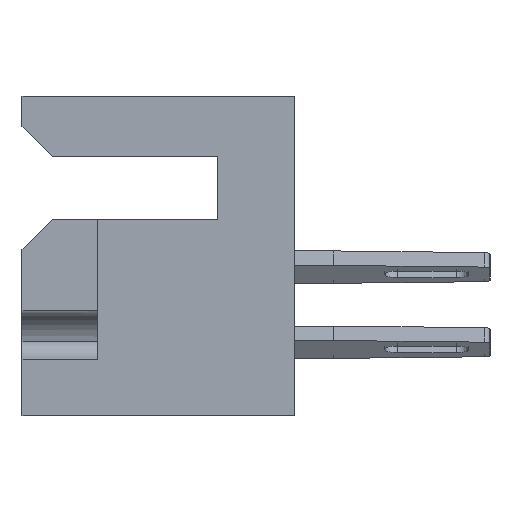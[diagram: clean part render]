
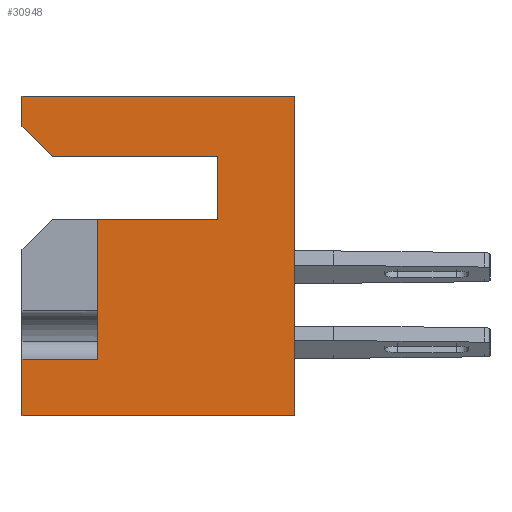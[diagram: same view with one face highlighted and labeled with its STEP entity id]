
A CAD part, left-side view. The second image highlights one B-rep face of the part: STEP entity #30948.
In plain terms, the highlighted planar face has unit normal (-1, 0, 0).
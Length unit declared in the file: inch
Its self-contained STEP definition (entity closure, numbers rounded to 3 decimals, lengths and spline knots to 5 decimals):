
#488 = EDGE_CURVE ( 'NONE', #5836, #26550, #2520, .T. ) ;
#700 = EDGE_CURVE ( 'NONE', #21298, #19477, #2494, .T. ) ;
#901 = LINE ( 'NONE', #11185, #5777 ) ;
#1414 = PLANE ( 'NONE',  #14213 ) ;
#1489 = DIRECTION ( 'NONE',  ( 0., 0., 1. ) ) ;
#1533 = ORIENTED_EDGE ( 'NONE', *, *, #700, .F. ) ;
#2153 = CARTESIAN_POINT ( 'NONE',  ( 0., 0.328, -0.205 ) ) ;
#2340 = DIRECTION ( 'NONE',  ( 0., 1., 0. ) ) ;
#2494 = LINE ( 'NONE', #4337, #11495 ) ;
#2520 = LINE ( 'NONE', #4237, #27203 ) ;
#3116 = CARTESIAN_POINT ( 'NONE',  ( 0., 0.128, -0.205 ) ) ;
#3589 = VERTEX_POINT ( 'NONE', #28175 ) ;
#4088 = CARTESIAN_POINT ( 'NONE',  ( 0., 0.453, 0. ) ) ;
#4125 = VERTEX_POINT ( 'NONE', #9381 ) ;
#4237 = CARTESIAN_POINT ( 'NONE',  ( 0., 0.128, -0.1 ) ) ;
#4260 = VECTOR ( 'NONE', #20819, 39.37008 ) ;
#4337 = CARTESIAN_POINT ( 'NONE',  ( 0., 0.453, 0. ) ) ;
#4658 = DIRECTION ( 'NONE',  ( 0., 0., 1. ) ) ;
#5777 = VECTOR ( 'NONE', #30473, 39.37008 ) ;
#5836 = VERTEX_POINT ( 'NONE', #18371 ) ;
#5914 = VERTEX_POINT ( 'NONE', #18853 ) ;
#6883 = LINE ( 'NONE', #22700, #22587 ) ;
#7056 = VECTOR ( 'NONE', #2340, 39.37008 ) ;
#7673 = EDGE_CURVE ( 'NONE', #17577, #4125, #25529, .T. ) ;
#8258 = ORIENTED_EDGE ( 'NONE', *, *, #13072, .F. ) ;
#8823 = ORIENTED_EDGE ( 'NONE', *, *, #28771, .T. ) ;
#9285 = EDGE_LOOP ( 'NONE', ( #25436, #1533, #11394, #15115, #19073, #30682, #8823, #24711, #25405, #24883, #8258 ) ) ;
#9306 = CARTESIAN_POINT ( 'NONE',  ( 0., 0.453, -0.437 ) ) ;
#9381 = CARTESIAN_POINT ( 'NONE',  ( 0., 0.453, 0. ) ) ;
#10070 = VECTOR ( 'NONE', #29678, 39.37008 ) ;
#10959 = DIRECTION ( 'NONE',  ( 0., 0., 1. ) ) ;
#11185 = CARTESIAN_POINT ( 'NONE',  ( 0., 0.328, -0.205 ) ) ;
#11394 = ORIENTED_EDGE ( 'NONE', *, *, #28670, .T. ) ;
#11495 = VECTOR ( 'NONE', #4658, 39.37008 ) ;
#11690 = EDGE_CURVE ( 'NONE', #26550, #3589, #13669, .T. ) ;
#12131 = VERTEX_POINT ( 'NONE', #26376 ) ;
#12239 = EDGE_CURVE ( 'NONE', #12131, #5914, #6883, .T. ) ;
#12410 = EDGE_CURVE ( 'NONE', #4125, #5914, #17750, .T. ) ;
#12455 = DIRECTION ( 'NONE',  ( 0., 0., 1. ) ) ;
#13072 = EDGE_CURVE ( 'NONE', #23057, #21686, #901, .T. ) ;
#13443 = CARTESIAN_POINT ( 'NONE',  ( 0., 0.453, 0. ) ) ;
#13669 = LINE ( 'NONE', #15216, #26010 ) ;
#14105 = EDGE_CURVE ( 'NONE', #5836, #21686, #23644, .T. ) ;
#14213 = AXIS2_PLACEMENT_3D ( 'NONE', #22846, #18183, #18483 ) ;
#15112 = DIRECTION ( 'NONE',  ( 0., 1., 0. ) ) ;
#15115 = ORIENTED_EDGE ( 'NONE', *, *, #12239, .T. ) ;
#15216 = CARTESIAN_POINT ( 'NONE',  ( 0., 0.128, -0.1 ) ) ;
#16727 = CARTESIAN_POINT ( 'NONE',  ( 0., 0.328, -0.437 ) ) ;
#17142 = LINE ( 'NONE', #18899, #7056 ) ;
#17577 = VERTEX_POINT ( 'NONE', #28411 ) ;
#17750 = LINE ( 'NONE', #4088, #4260 ) ;
#18183 = DIRECTION ( 'NONE',  ( 1., 0., 0. ) ) ;
#18371 = CARTESIAN_POINT ( 'NONE',  ( 0., 0.128, -0.205 ) ) ;
#18410 = CARTESIAN_POINT ( 'NONE',  ( 0., 0.403, -0.1 ) ) ;
#18483 = DIRECTION ( 'NONE',  ( 0., 0., -1. ) ) ;
#18853 = CARTESIAN_POINT ( 'NONE',  ( 0., 0., 0. ) ) ;
#18899 = CARTESIAN_POINT ( 'NONE',  ( 0., 0.328, -0.437 ) ) ;
#19073 = ORIENTED_EDGE ( 'NONE', *, *, #12410, .F. ) ;
#19477 = VERTEX_POINT ( 'NONE', #9306 ) ;
#20092 = CARTESIAN_POINT ( 'NONE',  ( 0., 0.453, -0.531 ) ) ;
#20819 = DIRECTION ( 'NONE',  ( 0., -1., 0. ) ) ;
#21298 = VERTEX_POINT ( 'NONE', #24364 ) ;
#21664 = LINE ( 'NONE', #20092, #10070 ) ;
#21686 = VERTEX_POINT ( 'NONE', #2153 ) ;
#22587 = VECTOR ( 'NONE', #12455, 39.37008 ) ;
#22700 = CARTESIAN_POINT ( 'NONE',  ( 0., 0., 0. ) ) ;
#22846 = CARTESIAN_POINT ( 'NONE',  ( 0., 0.453, 0. ) ) ;
#23057 = VERTEX_POINT ( 'NONE', #16727 ) ;
#23644 = LINE ( 'NONE', #3116, #28129 ) ;
#24364 = CARTESIAN_POINT ( 'NONE',  ( 0., 0.453, -0.531 ) ) ;
#24711 = ORIENTED_EDGE ( 'NONE', *, *, #11690, .F. ) ;
#24775 = DIRECTION ( 'NONE',  ( 0., 1., 0. ) ) ;
#24883 = ORIENTED_EDGE ( 'NONE', *, *, #14105, .T. ) ;
#25405 = ORIENTED_EDGE ( 'NONE', *, *, #488, .F. ) ;
#25436 = ORIENTED_EDGE ( 'NONE', *, *, #25667, .T. ) ;
#25529 = LINE ( 'NONE', #13443, #26633 ) ;
#25667 = EDGE_CURVE ( 'NONE', #23057, #19477, #17142, .T. ) ;
#26010 = VECTOR ( 'NONE', #15112, 39.37008 ) ;
#26376 = CARTESIAN_POINT ( 'NONE',  ( 0., 0., -0.531 ) ) ;
#26550 = VERTEX_POINT ( 'NONE', #28544 ) ;
#26633 = VECTOR ( 'NONE', #1489, 39.37008 ) ;
#26877 = VECTOR ( 'NONE', #30287, 39.37008 ) ;
#27203 = VECTOR ( 'NONE', #10959, 39.37008 ) ;
#27604 = LINE ( 'NONE', #18410, #26877 ) ;
#28129 = VECTOR ( 'NONE', #24775, 39.37008 ) ;
#28175 = CARTESIAN_POINT ( 'NONE',  ( 0., 0.403, -0.1 ) ) ;
#28411 = CARTESIAN_POINT ( 'NONE',  ( 0., 0.453, -0.05 ) ) ;
#28544 = CARTESIAN_POINT ( 'NONE',  ( 0., 0.128, -0.1 ) ) ;
#28579 = FACE_OUTER_BOUND ( 'NONE', #9285, .T. ) ;
#28670 = EDGE_CURVE ( 'NONE', #21298, #12131, #21664, .T. ) ;
#28771 = EDGE_CURVE ( 'NONE', #17577, #3589, #27604, .T. ) ;
#29678 = DIRECTION ( 'NONE',  ( 0., -1., 0. ) ) ;
#30287 = DIRECTION ( 'NONE',  ( 0., -0.707, -0.707 ) ) ;
#30473 = DIRECTION ( 'NONE',  ( 0., 0., 1. ) ) ;
#30682 = ORIENTED_EDGE ( 'NONE', *, *, #7673, .F. ) ;
#30948 = ADVANCED_FACE ( 'NONE', ( #28579 ), #1414, .F. ) ;
